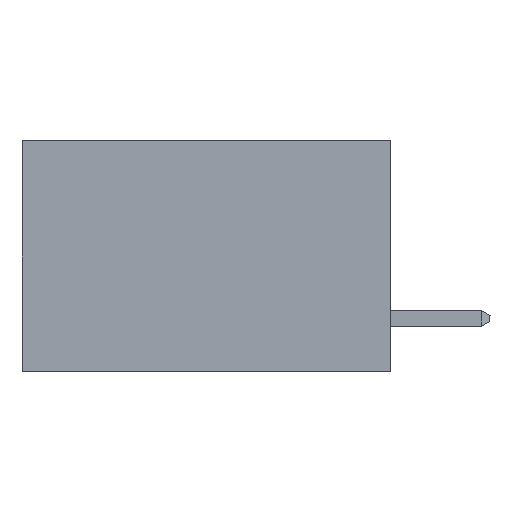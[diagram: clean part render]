
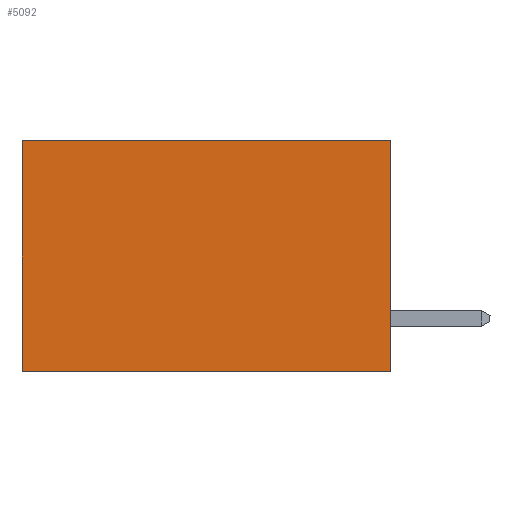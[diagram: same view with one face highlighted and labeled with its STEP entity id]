
A CAD part, left-side view. The second image highlights one B-rep face of the part: STEP entity #5092.
In plain terms, the highlighted planar face has unit normal (-1, 0, 0).
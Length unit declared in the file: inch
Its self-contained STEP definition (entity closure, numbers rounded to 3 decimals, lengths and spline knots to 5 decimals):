
#947 = DIRECTION ( 'NONE',  ( 0., 1., 0. ) ) ;
#965 = VECTOR ( 'NONE', #22695, 39.37008 ) ;
#3299 = CARTESIAN_POINT ( 'NONE',  ( 0.277, 0., 0. ) ) ;
#4293 = VECTOR ( 'NONE', #947, 39.37008 ) ;
#4908 = LINE ( 'NONE', #8839, #4293 ) ;
#5092 = ADVANCED_FACE ( 'NONE', ( #14444 ), #15262, .F. ) ;
#6899 = EDGE_LOOP ( 'NONE', ( #8695, #22404, #23920, #24084 ) ) ;
#7046 = CARTESIAN_POINT ( 'NONE',  ( 0.277, 0., -0.37 ) ) ;
#8044 = DIRECTION ( 'NONE',  ( 0., 0., -1. ) ) ;
#8065 = CARTESIAN_POINT ( 'NONE',  ( 0.277, 0., -0.37 ) ) ;
#8515 = EDGE_CURVE ( 'NONE', #22645, #13883, #11469, .T. ) ;
#8695 = ORIENTED_EDGE ( 'NONE', *, *, #18847, .T. ) ;
#8839 = CARTESIAN_POINT ( 'NONE',  ( 0.277, 0., -0.37 ) ) ;
#10269 = EDGE_CURVE ( 'NONE', #22645, #21801, #21218, .T. ) ;
#11469 = LINE ( 'NONE', #7046, #965 ) ;
#11910 = CARTESIAN_POINT ( 'NONE',  ( 0.277, 0.59, -0.37 ) ) ;
#12317 = VECTOR ( 'NONE', #8044, 39.37008 ) ;
#13317 = CARTESIAN_POINT ( 'NONE',  ( 0.277, 0.59, 0. ) ) ;
#13883 = VERTEX_POINT ( 'NONE', #8065 ) ;
#14444 = FACE_OUTER_BOUND ( 'NONE', #6899, .T. ) ;
#15262 = PLANE ( 'NONE',  #15901 ) ;
#15770 = VECTOR ( 'NONE', #19790, 39.37008 ) ;
#15901 = AXIS2_PLACEMENT_3D ( 'NONE', #16193, #17540, #18976 ) ;
#16193 = CARTESIAN_POINT ( 'NONE',  ( 0.277, 0., -0.37 ) ) ;
#16469 = EDGE_CURVE ( 'NONE', #13883, #17038, #4908, .T. ) ;
#17038 = VERTEX_POINT ( 'NONE', #22233 ) ;
#17540 = DIRECTION ( 'NONE',  ( 1., 0., 0. ) ) ;
#18240 = LINE ( 'NONE', #11910, #12317 ) ;
#18847 = EDGE_CURVE ( 'NONE', #21801, #17038, #18240, .T. ) ;
#18976 = DIRECTION ( 'NONE',  ( 0., 0., -1. ) ) ;
#19790 = DIRECTION ( 'NONE',  ( 0., 1., 0. ) ) ;
#21218 = LINE ( 'NONE', #23526, #15770 ) ;
#21801 = VERTEX_POINT ( 'NONE', #13317 ) ;
#22233 = CARTESIAN_POINT ( 'NONE',  ( 0.277, 0.59, -0.37 ) ) ;
#22404 = ORIENTED_EDGE ( 'NONE', *, *, #16469, .F. ) ;
#22645 = VERTEX_POINT ( 'NONE', #3299 ) ;
#22695 = DIRECTION ( 'NONE',  ( 0., 0., -1. ) ) ;
#23526 = CARTESIAN_POINT ( 'NONE',  ( 0.277, 0., 0. ) ) ;
#23920 = ORIENTED_EDGE ( 'NONE', *, *, #8515, .F. ) ;
#24084 = ORIENTED_EDGE ( 'NONE', *, *, #10269, .T. ) ;
